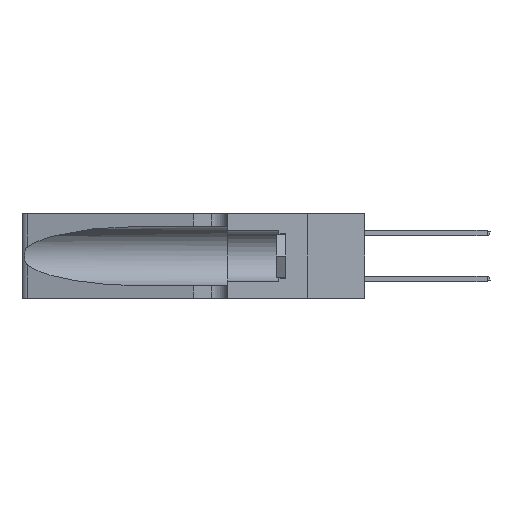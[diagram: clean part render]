
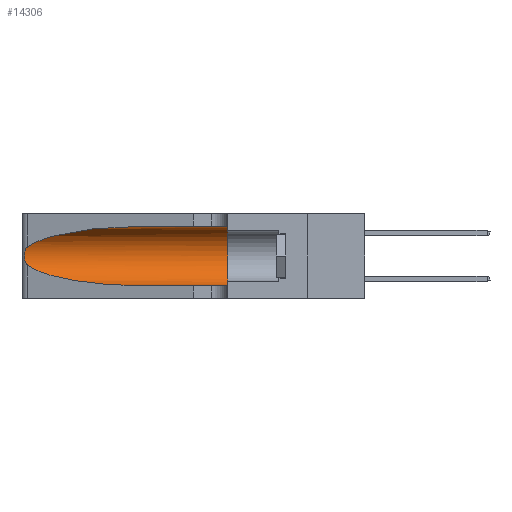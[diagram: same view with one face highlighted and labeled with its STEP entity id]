
A CAD part, left-side view. The second image highlights one B-rep face of the part: STEP entity #14306.
In plain terms, the highlighted cylindrical face has radius 3.308 mm (diameter 6.617 mm), a partial arc.
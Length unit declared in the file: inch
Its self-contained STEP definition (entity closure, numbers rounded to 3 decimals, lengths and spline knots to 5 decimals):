
#228 = CARTESIAN_POINT ( 'NONE',  ( 0.26075, 1.23896, 0.19203 ) ) ;
#906 = VECTOR ( 'NONE', #12299, 39.37008 ) ;
#2342 = CARTESIAN_POINT ( 'NONE',  ( 0.1305, 0.72297, 0.05475 ) ) ;
#3084 = CARTESIAN_POINT ( 'NONE',  ( 0.26017, 1.23833, 0.17102 ) ) ;
#4061 = VECTOR ( 'NONE', #30392, 39.37008 ) ;
#4438 = CARTESIAN_POINT ( 'NONE',  ( 0.25487, 1.22718, 0.14631 ) ) ;
#4590 = DIRECTION ( 'NONE',  ( 0., -1., 0. ) ) ;
#4767 = CARTESIAN_POINT ( 'NONE',  ( 0.1305, 0.35, 0.31525 ) ) ;
#5891 = EDGE_CURVE ( 'NONE', #26161, #15328, #29159, .T. ) ;
#5904 = CARTESIAN_POINT ( 'NONE',  ( 0.25789, 1.23486, 0.15765 ) ) ;
#6994 = EDGE_CURVE ( 'NONE', #26161, #30738, #32677, .T. ) ;
#7118 = CARTESIAN_POINT ( 'NONE',  ( 0.1305, 0.35, 0.185 ) ) ;
#7867 = FACE_OUTER_BOUND ( 'NONE', #13598, .T. ) ;
#8752 = CARTESIAN_POINT ( 'NONE',  ( 0.25555, 1.22993, 0.14849 ) ) ;
#9033 = ORIENTED_EDGE ( 'NONE', *, *, #17333, .T. ) ;
#9975 = DIRECTION ( 'NONE',  ( 0., 0., 1. ) ) ;
#10697 = CARTESIAN_POINT ( 'NONE',  ( 0.1305, 1.61858, 0.05475 ) ) ;
#12299 = DIRECTION ( 'NONE',  ( 0., -1., 0. ) ) ;
#12558 = CARTESIAN_POINT ( 'NONE',  ( 0.1305, 0.35, 0.05475 ) ) ;
#13530 = VERTEX_POINT ( 'NONE', #12558 ) ;
#13598 = EDGE_LOOP ( 'NONE', ( #34054, #27090, #21579, #9033, #29407, #23214 ) ) ;
#14306 = ADVANCED_FACE ( 'NONE', ( #7867 ), #14572, .F. ) ;
#14369 = CARTESIAN_POINT ( 'NONE',  ( 0.25787, 1.23484, 0.2124 ) ) ;
#14572 = CYLINDRICAL_SURFACE ( 'NONE', #14982, 0.13025 ) ;
#14982 = AXIS2_PLACEMENT_3D ( 'NONE', #24387, #4590, #15920 ) ;
#15328 = VERTEX_POINT ( 'NONE', #4767 ) ;
#15920 = DIRECTION ( 'NONE',  ( 0., 0., -1. ) ) ;
#16117 = CARTESIAN_POINT ( 'NONE',  ( 0.1305, 0.72297, 0.31525 ) ) ;
#16847 = CIRCLE ( 'NONE', #24739, 0.13025 ) ;
#17014 = B_SPLINE_CURVE_WITH_KNOTS ( 'NONE', 3,
 ( #28372, #19987, #31179, #14369, #33967, #17274, #228, #20100, #3084, #22911, #5904, #25714, #8752, #28496 ),
 .UNSPECIFIED., .F., .F.,
 ( 4, 2, 2, 2, 2, 2, 4 ),
 ( 0., 0.00027, 0.00053, 0.00107, 0.0016, 0.00187, 0.00214 ),
 .UNSPECIFIED. ) ;
#17274 = CARTESIAN_POINT ( 'NONE',  ( 0.26018, 1.23835, 0.19895 ) ) ;
#17333 = EDGE_CURVE ( 'NONE', #23388, #13530, #18315, .T. ) ;
#18315 = LINE ( 'NONE', #10697, #4061 ) ;
#18968 = EDGE_CURVE ( 'NONE', #15328, #13530, #16847, .T. ) ;
#19367 = CARTESIAN_POINT ( 'NONE',  ( 0.18966, 0.96281, 0.05475 ) ) ;
#19987 = CARTESIAN_POINT ( 'NONE',  ( 0.25555, 1.22994, 0.2215 ) ) ;
#20100 = CARTESIAN_POINT ( 'NONE',  ( 0.26075, 1.23896, 0.178 ) ) ;
#21579 = ORIENTED_EDGE ( 'NONE', *, *, #27919, .T. ) ;
#22911 = CARTESIAN_POINT ( 'NONE',  ( 0.25856, 1.23593, 0.16098 ) ) ;
#23022 = CARTESIAN_POINT ( 'NONE',  ( 0.1305, 0.72297, 0.31525 ) ) ;
#23214 = ORIENTED_EDGE ( 'NONE', *, *, #5891, .F. ) ;
#23388 = VERTEX_POINT ( 'NONE', #27127 ) ;
#23529 =( BOUNDED_CURVE ( )  B_SPLINE_CURVE ( 3, ( #27650, #30448, #19367, #2342 ),
 .UNSPECIFIED., .F., .F. ) 
 B_SPLINE_CURVE_WITH_KNOTS ( ( 4, 4 ),
 ( 3.44316, 4.71239 ),
 .UNSPECIFIED. ) 
 CURVE ( )  GEOMETRIC_REPRESENTATION_ITEM ( )  RATIONAL_B_SPLINE_CURVE ( ( 1., 0.87, 0.87, 1. ) ) 
 REPRESENTATION_ITEM ( '' )  );
#24271 = CARTESIAN_POINT ( 'NONE',  ( 0.25487, 1.22718, 0.22369 ) ) ;
#24387 = CARTESIAN_POINT ( 'NONE',  ( 0.1305, 1.61858, 0.185 ) ) ;
#24739 = AXIS2_PLACEMENT_3D ( 'NONE', #7118, #26897, #9975 ) ;
#25714 = CARTESIAN_POINT ( 'NONE',  ( 0.25639, 1.23186, 0.15144 ) ) ;
#26161 = VERTEX_POINT ( 'NONE', #16117 ) ;
#26897 = DIRECTION ( 'NONE',  ( 0., 1., 0. ) ) ;
#27090 = ORIENTED_EDGE ( 'NONE', *, *, #31058, .T. ) ;
#27127 = CARTESIAN_POINT ( 'NONE',  ( 0.1305, 0.72297, 0.05475 ) ) ;
#27650 = CARTESIAN_POINT ( 'NONE',  ( 0.25487, 1.22718, 0.14631 ) ) ;
#27919 = EDGE_CURVE ( 'NONE', #28310, #23388, #23529, .T. ) ;
#28310 = VERTEX_POINT ( 'NONE', #4438 ) ;
#28372 = CARTESIAN_POINT ( 'NONE',  ( 0.25487, 1.22718, 0.22369 ) ) ;
#28496 = CARTESIAN_POINT ( 'NONE',  ( 0.25487, 1.22718, 0.14631 ) ) ;
#28602 = CARTESIAN_POINT ( 'NONE',  ( 0.18966, 0.96281, 0.31525 ) ) ;
#29159 = LINE ( 'NONE', #29165, #906 ) ;
#29165 = CARTESIAN_POINT ( 'NONE',  ( 0.1305, 1.61858, 0.31525 ) ) ;
#29407 = ORIENTED_EDGE ( 'NONE', *, *, #18968, .F. ) ;
#30392 = DIRECTION ( 'NONE',  ( 0., -1., 0. ) ) ;
#30448 = CARTESIAN_POINT ( 'NONE',  ( 0.2373, 1.15595, 0.08982 ) ) ;
#30738 = VERTEX_POINT ( 'NONE', #24271 ) ;
#31058 = EDGE_CURVE ( 'NONE', #30738, #28310, #17014, .T. ) ;
#31179 = CARTESIAN_POINT ( 'NONE',  ( 0.25639, 1.23184, 0.21858 ) ) ;
#31408 = CARTESIAN_POINT ( 'NONE',  ( 0.2373, 1.15595, 0.28018 ) ) ;
#32677 =( BOUNDED_CURVE ( )  B_SPLINE_CURVE ( 3, ( #23022, #28602, #31408, #34203 ),
 .UNSPECIFIED., .F., .F. ) 
 B_SPLINE_CURVE_WITH_KNOTS ( ( 4, 4 ),
 ( 1.5708, 2.84003 ),
 .UNSPECIFIED. ) 
 CURVE ( )  GEOMETRIC_REPRESENTATION_ITEM ( )  RATIONAL_B_SPLINE_CURVE ( ( 1., 0.87, 0.87, 1. ) ) 
 REPRESENTATION_ITEM ( '' )  );
#33967 = CARTESIAN_POINT ( 'NONE',  ( 0.25854, 1.2359, 0.20912 ) ) ;
#34054 = ORIENTED_EDGE ( 'NONE', *, *, #6994, .T. ) ;
#34203 = CARTESIAN_POINT ( 'NONE',  ( 0.25487, 1.22718, 0.22369 ) ) ;
